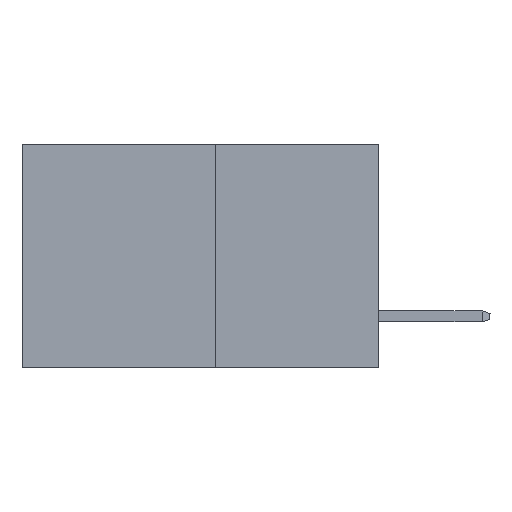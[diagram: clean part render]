
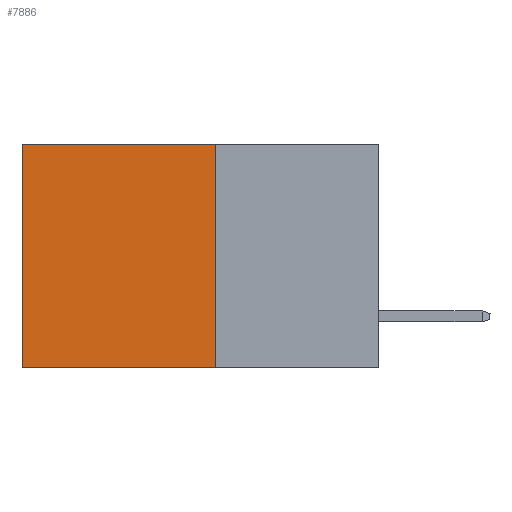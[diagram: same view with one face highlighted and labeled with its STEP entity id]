
A CAD part, left-side view. The second image highlights one B-rep face of the part: STEP entity #7886.
In plain terms, the highlighted planar face has unit normal (-1, 0, 0).
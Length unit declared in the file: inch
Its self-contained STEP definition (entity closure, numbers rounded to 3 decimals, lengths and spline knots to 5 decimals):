
#186 = VERTEX_POINT ( 'NONE', #8146 ) ;
#253 = VECTOR ( 'NONE', #3975, 39.37008 ) ;
#466 = CARTESIAN_POINT ( 'NONE',  ( 0.277, 0.59, -0.37 ) ) ;
#1305 = FACE_OUTER_BOUND ( 'NONE', #4553, .T. ) ;
#1311 = EDGE_CURVE ( 'NONE', #1897, #4043, #5922, .T. ) ;
#1517 = PLANE ( 'NONE',  #6967 ) ;
#1634 = VECTOR ( 'NONE', #7114, 39.37008 ) ;
#1897 = VERTEX_POINT ( 'NONE', #4347 ) ;
#2221 = VERTEX_POINT ( 'NONE', #6071 ) ;
#2358 = CARTESIAN_POINT ( 'NONE',  ( 0.277, 0.27, -0.37 ) ) ;
#2746 = DIRECTION ( 'NONE',  ( 0., 0., -1. ) ) ;
#3002 = CARTESIAN_POINT ( 'NONE',  ( 0.277, 0.27, -0.37 ) ) ;
#3640 = CARTESIAN_POINT ( 'NONE',  ( 0.277, 0.27, -0.37 ) ) ;
#3860 = ORIENTED_EDGE ( 'NONE', *, *, #8022, .T. ) ;
#3975 = DIRECTION ( 'NONE',  ( 0., 1., 0. ) ) ;
#4043 = VERTEX_POINT ( 'NONE', #2358 ) ;
#4347 = CARTESIAN_POINT ( 'NONE',  ( 0.277, 0.27, 0. ) ) ;
#4553 = EDGE_LOOP ( 'NONE', ( #6985, #6145, #6141, #3860 ) ) ;
#4675 = DIRECTION ( 'NONE',  ( 0., 0., -1. ) ) ;
#5042 = CARTESIAN_POINT ( 'NONE',  ( 0.277, 0.27, -0.37 ) ) ;
#5732 = LINE ( 'NONE', #6852, #253 ) ;
#5922 = LINE ( 'NONE', #3002, #7478 ) ;
#6071 = CARTESIAN_POINT ( 'NONE',  ( 0.277, 0.59, 0. ) ) ;
#6141 = ORIENTED_EDGE ( 'NONE', *, *, #1311, .F. ) ;
#6145 = ORIENTED_EDGE ( 'NONE', *, *, #6192, .F. ) ;
#6192 = EDGE_CURVE ( 'NONE', #4043, #186, #6794, .T. ) ;
#6605 = LINE ( 'NONE', #466, #8165 ) ;
#6625 = EDGE_CURVE ( 'NONE', #2221, #186, #6605, .T. ) ;
#6794 = LINE ( 'NONE', #5042, #1634 ) ;
#6852 = CARTESIAN_POINT ( 'NONE',  ( 0.277, 0.27, 0. ) ) ;
#6967 = AXIS2_PLACEMENT_3D ( 'NONE', #3640, #7709, #7703 ) ;
#6985 = ORIENTED_EDGE ( 'NONE', *, *, #6625, .T. ) ;
#7114 = DIRECTION ( 'NONE',  ( 0., 1., 0. ) ) ;
#7478 = VECTOR ( 'NONE', #2746, 39.37008 ) ;
#7703 = DIRECTION ( 'NONE',  ( 0., 0., -1. ) ) ;
#7709 = DIRECTION ( 'NONE',  ( 1., 0., 0. ) ) ;
#7886 = ADVANCED_FACE ( 'NONE', ( #1305 ), #1517, .F. ) ;
#8022 = EDGE_CURVE ( 'NONE', #1897, #2221, #5732, .T. ) ;
#8146 = CARTESIAN_POINT ( 'NONE',  ( 0.277, 0.59, -0.37 ) ) ;
#8165 = VECTOR ( 'NONE', #4675, 39.37008 ) ;
